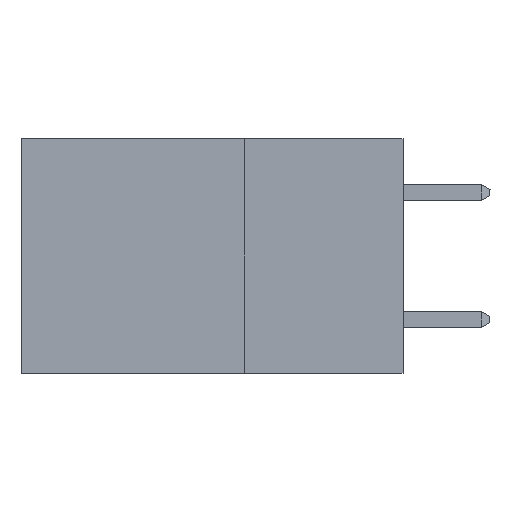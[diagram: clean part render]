
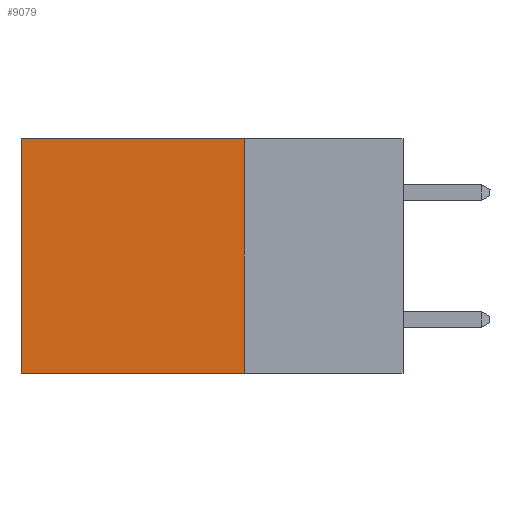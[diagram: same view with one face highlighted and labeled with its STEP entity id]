
A CAD part, left-side view. The second image highlights one B-rep face of the part: STEP entity #9079.
In plain terms, the highlighted planar face has unit normal (-1, 0, 0).
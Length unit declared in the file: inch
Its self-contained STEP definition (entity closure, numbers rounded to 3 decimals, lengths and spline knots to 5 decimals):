
#2012 = DIRECTION ( 'NONE',  ( 1., 0., 0. ) ) ;
#2087 = DIRECTION ( 'NONE',  ( 0., 1., 0. ) ) ;
#2176 = VERTEX_POINT ( 'NONE', #21512 ) ;
#2274 = EDGE_CURVE ( 'NONE', #12190, #10371, #26701, .T. ) ;
#3890 = LINE ( 'NONE', #18431, #15912 ) ;
#5836 = CARTESIAN_POINT ( 'NONE',  ( 0.2875, 0.25, 0. ) ) ;
#6272 = DIRECTION ( 'NONE',  ( 0., 1., 0. ) ) ;
#6337 = VERTEX_POINT ( 'NONE', #5836 ) ;
#6674 = LINE ( 'NONE', #13370, #15275 ) ;
#9079 = ADVANCED_FACE ( 'NONE', ( #26058 ), #18578, .F. ) ;
#10371 = VERTEX_POINT ( 'NONE', #23223 ) ;
#10999 = VECTOR ( 'NONE', #2087, 39.37008 ) ;
#11632 = CARTESIAN_POINT ( 'NONE',  ( 0.2875, 0.25, -0.37 ) ) ;
#12190 = VERTEX_POINT ( 'NONE', #27167 ) ;
#13370 = CARTESIAN_POINT ( 'NONE',  ( 0.2875, 0.25, 0. ) ) ;
#14334 = EDGE_LOOP ( 'NONE', ( #17896, #30272, #22921, #23199 ) ) ;
#14965 = EDGE_CURVE ( 'NONE', #6337, #2176, #3890, .T. ) ;
#15275 = VECTOR ( 'NONE', #18163, 39.37008 ) ;
#15912 = VECTOR ( 'NONE', #6272, 39.37008 ) ;
#16076 = CARTESIAN_POINT ( 'NONE',  ( 0.2875, 0.6, 0. ) ) ;
#17896 = ORIENTED_EDGE ( 'NONE', *, *, #28569, .T. ) ;
#18163 = DIRECTION ( 'NONE',  ( 0., 0., -1. ) ) ;
#18431 = CARTESIAN_POINT ( 'NONE',  ( 0.2875, 0.25, 0. ) ) ;
#18480 = DIRECTION ( 'NONE',  ( 0., 0., -1. ) ) ;
#18560 = AXIS2_PLACEMENT_3D ( 'NONE', #27974, #2012, #18674 ) ;
#18578 = PLANE ( 'NONE',  #18560 ) ;
#18674 = DIRECTION ( 'NONE',  ( 0., 0., -1. ) ) ;
#21512 = CARTESIAN_POINT ( 'NONE',  ( 0.2875, 0.6, 0. ) ) ;
#21943 = LINE ( 'NONE', #16076, #27566 ) ;
#22921 = ORIENTED_EDGE ( 'NONE', *, *, #30758, .F. ) ;
#23199 = ORIENTED_EDGE ( 'NONE', *, *, #14965, .T. ) ;
#23223 = CARTESIAN_POINT ( 'NONE',  ( 0.2875, 0.6, -0.37 ) ) ;
#26058 = FACE_OUTER_BOUND ( 'NONE', #14334, .T. ) ;
#26701 = LINE ( 'NONE', #11632, #10999 ) ;
#27167 = CARTESIAN_POINT ( 'NONE',  ( 0.2875, 0.25, -0.37 ) ) ;
#27566 = VECTOR ( 'NONE', #18480, 39.37008 ) ;
#27974 = CARTESIAN_POINT ( 'NONE',  ( 0.2875, 0.25, 0. ) ) ;
#28569 = EDGE_CURVE ( 'NONE', #2176, #10371, #21943, .T. ) ;
#30272 = ORIENTED_EDGE ( 'NONE', *, *, #2274, .F. ) ;
#30758 = EDGE_CURVE ( 'NONE', #6337, #12190, #6674, .T. ) ;
